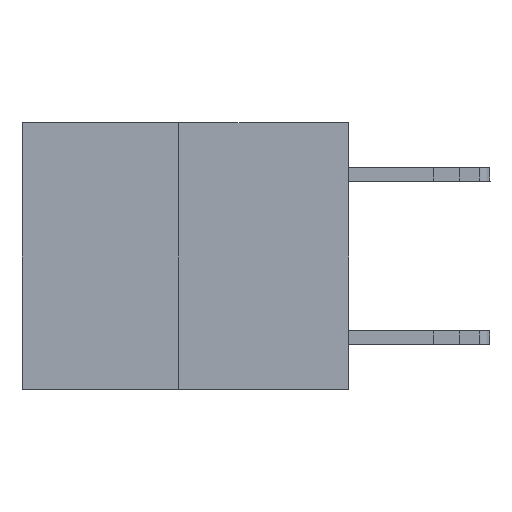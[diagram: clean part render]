
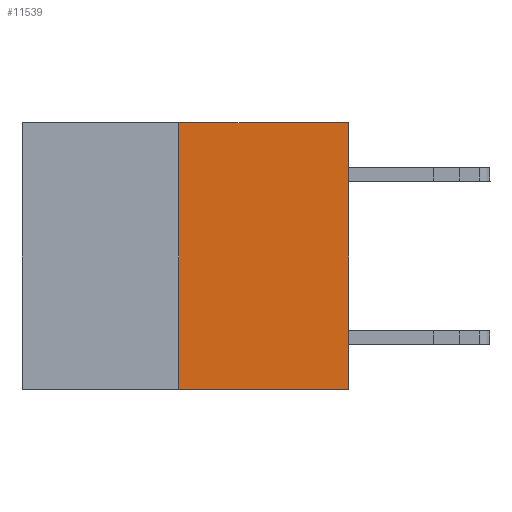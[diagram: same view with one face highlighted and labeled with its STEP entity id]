
A CAD part, left-side view. The second image highlights one B-rep face of the part: STEP entity #11539.
In plain terms, the highlighted planar face has unit normal (-1, 0, 0).
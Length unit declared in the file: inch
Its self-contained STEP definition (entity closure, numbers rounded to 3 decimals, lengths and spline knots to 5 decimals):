
#410 = DIRECTION ( 'NONE',  ( 1., 0., 0. ) ) ;
#717 = VERTEX_POINT ( 'NONE', #1398 ) ;
#795 = CARTESIAN_POINT ( 'NONE',  ( 0., 0.6, -0.49 ) ) ;
#956 = VECTOR ( 'NONE', #19913, 39.37008 ) ;
#1398 = CARTESIAN_POINT ( 'NONE',  ( 0., 0.312, 0. ) ) ;
#1419 = DIRECTION ( 'NONE',  ( 0., 0., 1. ) ) ;
#1805 = ORIENTED_EDGE ( 'NONE', *, *, #23107, .F. ) ;
#2904 = CARTESIAN_POINT ( 'NONE',  ( 0., 0.6, 0. ) ) ;
#2973 = EDGE_CURVE ( 'NONE', #9570, #7699, #25584, .T. ) ;
#2999 = DIRECTION ( 'NONE',  ( 0., -1., 0. ) ) ;
#4473 = CARTESIAN_POINT ( 'NONE',  ( 0., 0., 0. ) ) ;
#4486 = EDGE_CURVE ( 'NONE', #15263, #9570, #6806, .T. ) ;
#6677 = DIRECTION ( 'NONE',  ( 0., 0., -1. ) ) ;
#6711 = LINE ( 'NONE', #2904, #956 ) ;
#6806 = LINE ( 'NONE', #795, #11524 ) ;
#7426 = ORIENTED_EDGE ( 'NONE', *, *, #4486, .T. ) ;
#7588 = DIRECTION ( 'NONE',  ( 0., 0., 1. ) ) ;
#7699 = VERTEX_POINT ( 'NONE', #4473 ) ;
#9570 = VERTEX_POINT ( 'NONE', #11059 ) ;
#10150 = EDGE_CURVE ( 'NONE', #717, #7699, #6711, .T. ) ;
#11059 = CARTESIAN_POINT ( 'NONE',  ( 0., 0., -0.49 ) ) ;
#11194 = ORIENTED_EDGE ( 'NONE', *, *, #10150, .F. ) ;
#11524 = VECTOR ( 'NONE', #2999, 39.37008 ) ;
#11539 = ADVANCED_FACE ( 'NONE', ( #12661 ), #26461, .F. ) ;
#11562 = CARTESIAN_POINT ( 'NONE',  ( 0., 0.312, -0.49 ) ) ;
#12661 = FACE_OUTER_BOUND ( 'NONE', #23201, .T. ) ;
#13547 = LINE ( 'NONE', #11562, #19981 ) ;
#14201 = ORIENTED_EDGE ( 'NONE', *, *, #2973, .T. ) ;
#15263 = VERTEX_POINT ( 'NONE', #15282 ) ;
#15282 = CARTESIAN_POINT ( 'NONE',  ( 0., 0.312, -0.49 ) ) ;
#15837 = AXIS2_PLACEMENT_3D ( 'NONE', #19827, #410, #6677 ) ;
#19827 = CARTESIAN_POINT ( 'NONE',  ( 0., 0.6, 0. ) ) ;
#19913 = DIRECTION ( 'NONE',  ( 0., -1., 0. ) ) ;
#19981 = VECTOR ( 'NONE', #1419, 39.37008 ) ;
#23107 = EDGE_CURVE ( 'NONE', #15263, #717, #13547, .T. ) ;
#23201 = EDGE_LOOP ( 'NONE', ( #1805, #7426, #14201, #11194 ) ) ;
#23526 = VECTOR ( 'NONE', #7588, 39.37008 ) ;
#24898 = CARTESIAN_POINT ( 'NONE',  ( 0., 0., 0. ) ) ;
#25584 = LINE ( 'NONE', #24898, #23526 ) ;
#26461 = PLANE ( 'NONE',  #15837 ) ;
